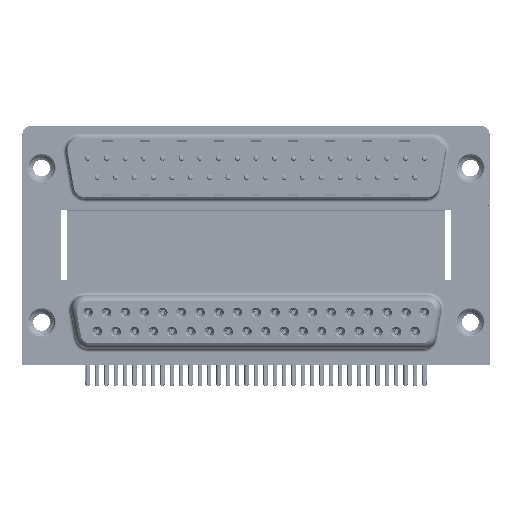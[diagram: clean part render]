
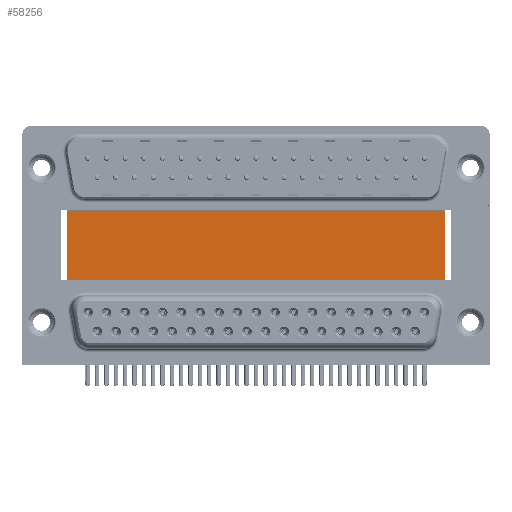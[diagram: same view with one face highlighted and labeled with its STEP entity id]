
A CAD part, top view. The second image highlights one B-rep face of the part: STEP entity #58256.
In plain terms, the highlighted planar face has unit normal (0, 0, 1).
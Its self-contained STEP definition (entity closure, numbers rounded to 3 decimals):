
#2862 = DIRECTION ( 'NONE',  ( 1., 0., 0. ) ) ;
#3433 = ORIENTED_EDGE ( 'NONE', *, *, #6919, .T. ) ;
#3490 = FACE_OUTER_BOUND ( 'NONE', #67252, .T. ) ;
#6919 = EDGE_CURVE ( 'NONE', #10767, #38975, #54637, .T. ) ;
#7742 = CARTESIAN_POINT ( 'NONE',  ( 3.79, 16.585, -12. ) ) ;
#8654 = LINE ( 'NONE', #60355, #18540 ) ;
#9611 = CARTESIAN_POINT ( 'NONE',  ( 3.79, 16.585, -12. ) ) ;
#10767 = VERTEX_POINT ( 'NONE', #9611 ) ;
#11970 = CARTESIAN_POINT ( 'NONE',  ( 3.79, -3.735, -12. ) ) ;
#16244 = VECTOR ( 'NONE', #43019, 1000. ) ;
#16497 = ORIENTED_EDGE ( 'NONE', *, *, #39869, .F. ) ;
#17325 = VECTOR ( 'NONE', #35198, 1000. ) ;
#18540 = VECTOR ( 'NONE', #54206, 1000. ) ;
#18598 = DIRECTION ( 'NONE',  ( -1., 0., 0. ) ) ;
#18933 = PLANE ( 'NONE',  #32970 ) ;
#19281 = CARTESIAN_POINT ( 'NONE',  ( 3.79, 16.585, -12. ) ) ;
#24940 = CARTESIAN_POINT ( 'NONE',  ( 59.71, 16.585, -12. ) ) ;
#32970 = AXIS2_PLACEMENT_3D ( 'NONE', #19281, #56205, #18598 ) ;
#35198 = DIRECTION ( 'NONE',  ( 0., -1., 0. ) ) ;
#38467 = VERTEX_POINT ( 'NONE', #48343 ) ;
#38975 = VERTEX_POINT ( 'NONE', #11970 ) ;
#39869 = EDGE_CURVE ( 'NONE', #10767, #52616, #54881, .T. ) ;
#40622 = ORIENTED_EDGE ( 'NONE', *, *, #42726, .F. ) ;
#42726 = EDGE_CURVE ( 'NONE', #52616, #38467, #55723, .T. ) ;
#43019 = DIRECTION ( 'NONE',  ( 0., -1., 0. ) ) ;
#44959 = CARTESIAN_POINT ( 'NONE',  ( 3.79, 16.585, -12. ) ) ;
#45717 = EDGE_CURVE ( 'NONE', #38975, #38467, #8654, .T. ) ;
#46859 = CARTESIAN_POINT ( 'NONE',  ( 59.71, 16.585, -12. ) ) ;
#48343 = CARTESIAN_POINT ( 'NONE',  ( 59.71, -3.735, -12. ) ) ;
#51433 = VECTOR ( 'NONE', #2862, 1000. ) ;
#52616 = VERTEX_POINT ( 'NONE', #46859 ) ;
#54206 = DIRECTION ( 'NONE',  ( 1., 0., 0. ) ) ;
#54637 = LINE ( 'NONE', #7742, #16244 ) ;
#54881 = LINE ( 'NONE', #44959, #51433 ) ;
#55723 = LINE ( 'NONE', #24940, #17325 ) ;
#56205 = DIRECTION ( 'NONE',  ( 0., 0., -1. ) ) ;
#58256 = ADVANCED_FACE ( 'NONE', ( #3490 ), #18933, .F. ) ;
#60355 = CARTESIAN_POINT ( 'NONE',  ( 3.79, -3.735, -12. ) ) ;
#66005 = ORIENTED_EDGE ( 'NONE', *, *, #45717, .T. ) ;
#67252 = EDGE_LOOP ( 'NONE', ( #66005, #40622, #16497, #3433 ) ) ;
